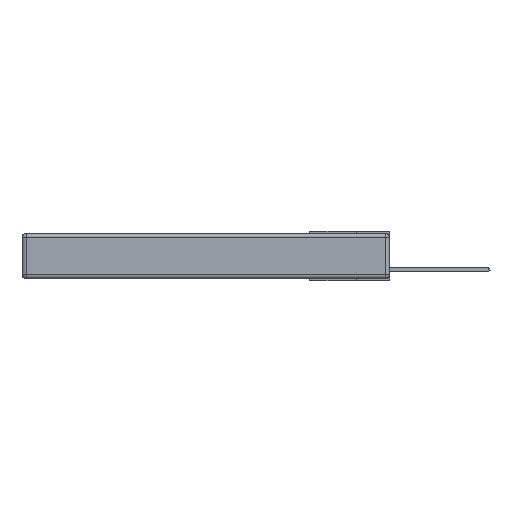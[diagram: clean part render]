
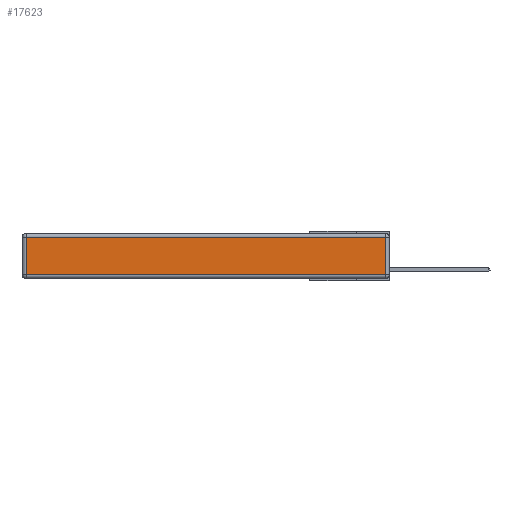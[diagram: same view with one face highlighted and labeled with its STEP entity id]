
A CAD part, left-side view. The second image highlights one B-rep face of the part: STEP entity #17623.
In plain terms, the highlighted planar face has unit normal (-1, 0, 0).
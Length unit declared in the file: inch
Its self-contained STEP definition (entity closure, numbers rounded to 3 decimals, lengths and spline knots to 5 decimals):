
#166 = ORIENTED_EDGE ( 'NONE', *, *, #10997, .T. ) ;
#874 = LINE ( 'NONE', #17231, #4867 ) ;
#1674 = DIRECTION ( 'NONE',  ( -1., 0., 0. ) ) ;
#1753 = LINE ( 'NONE', #15597, #8483 ) ;
#2116 = DIRECTION ( 'NONE',  ( 0., 0., 1. ) ) ;
#2444 = CARTESIAN_POINT ( 'NONE',  ( 0., 2.72, -0.313 ) ) ;
#2800 = VECTOR ( 'NONE', #17103, 39.37008 ) ;
#2832 = CARTESIAN_POINT ( 'NONE',  ( 0., 2.72, -0.03 ) ) ;
#3470 = DIRECTION ( 'NONE',  ( 0., 0., -1. ) ) ;
#4132 = LINE ( 'NONE', #11708, #10312 ) ;
#4867 = VECTOR ( 'NONE', #3470, 39.37008 ) ;
#5329 = EDGE_LOOP ( 'NONE', ( #12368, #16804, #7585, #166 ) ) ;
#6105 = AXIS2_PLACEMENT_3D ( 'NONE', #8236, #1674, #8301 ) ;
#6226 = VERTEX_POINT ( 'NONE', #2832 ) ;
#6790 = PLANE ( 'NONE',  #6105 ) ;
#7585 = ORIENTED_EDGE ( 'NONE', *, *, #15334, .T. ) ;
#7932 = VERTEX_POINT ( 'NONE', #2444 ) ;
#8236 = CARTESIAN_POINT ( 'NONE',  ( 0., 0., -0.343 ) ) ;
#8301 = DIRECTION ( 'NONE',  ( 0., 0., 1. ) ) ;
#8483 = VECTOR ( 'NONE', #2116, 39.37008 ) ;
#8772 = CARTESIAN_POINT ( 'NONE',  ( 0., 2.75, -0.03 ) ) ;
#9564 = CARTESIAN_POINT ( 'NONE',  ( 0., 0.03, -0.313 ) ) ;
#9842 = EDGE_CURVE ( 'NONE', #7932, #18884, #4132, .T. ) ;
#10122 = CARTESIAN_POINT ( 'NONE',  ( 0., 0.03, -0.03 ) ) ;
#10312 = VECTOR ( 'NONE', #21802, 39.37008 ) ;
#10997 = EDGE_CURVE ( 'NONE', #6226, #7932, #874, .T. ) ;
#11708 = CARTESIAN_POINT ( 'NONE',  ( 0., 0., -0.313 ) ) ;
#12368 = ORIENTED_EDGE ( 'NONE', *, *, #9842, .T. ) ;
#12524 = FACE_OUTER_BOUND ( 'NONE', #5329, .T. ) ;
#14638 = EDGE_CURVE ( 'NONE', #18884, #16541, #1753, .T. ) ;
#15334 = EDGE_CURVE ( 'NONE', #16541, #6226, #15368, .T. ) ;
#15368 = LINE ( 'NONE', #8772, #2800 ) ;
#15597 = CARTESIAN_POINT ( 'NONE',  ( 0., 0.03, -0.343 ) ) ;
#16541 = VERTEX_POINT ( 'NONE', #10122 ) ;
#16804 = ORIENTED_EDGE ( 'NONE', *, *, #14638, .T. ) ;
#17103 = DIRECTION ( 'NONE',  ( 0., 1., 0. ) ) ;
#17231 = CARTESIAN_POINT ( 'NONE',  ( 0., 2.72, -0.343 ) ) ;
#17623 = ADVANCED_FACE ( 'NONE', ( #12524 ), #6790, .T. ) ;
#18884 = VERTEX_POINT ( 'NONE', #9564 ) ;
#21802 = DIRECTION ( 'NONE',  ( 0., -1., 0. ) ) ;
